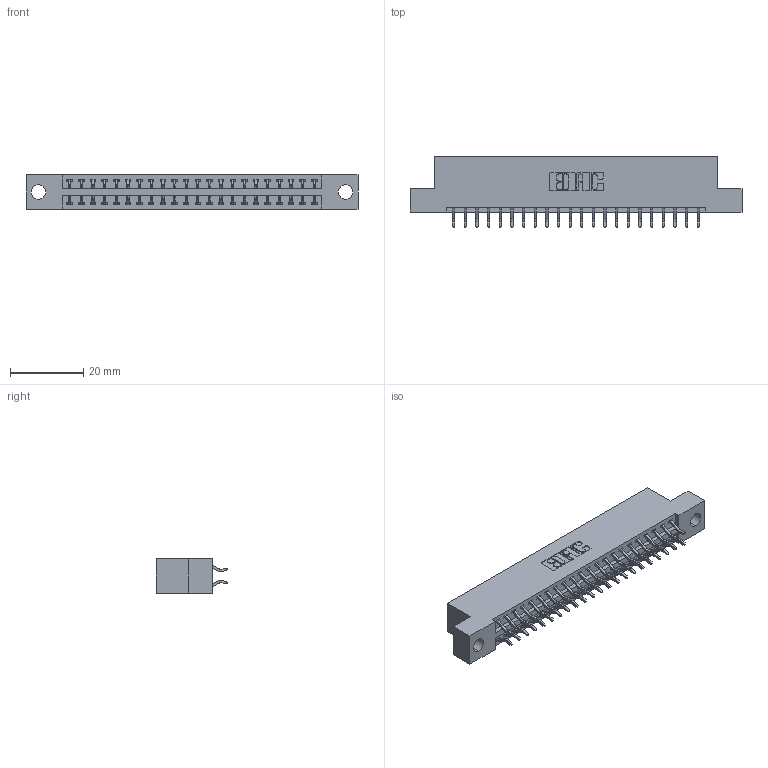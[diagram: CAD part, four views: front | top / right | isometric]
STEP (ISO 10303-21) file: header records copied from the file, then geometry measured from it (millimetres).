
FILE_DESCRIPTION (( 'STEP AP203' ), '1' );
FILE_NAME ('346-044-556-204.STEP', '2022-05-20T07:50:15', ( '' ), ( '' ), 'SwSTEP 2.0', 'SolidWorks 2020', '' );
FILE_SCHEMA (( 'CONFIG_CONTROL_DESIGN' ));
Length unit declared in the file: inch
Products named in the file (3): 345-292-001_556 Tail; 346-044-556-204; 346 Part_Flush Mounting Lugs - 0.156 Dia-TH
Assembly tree (45 placements, depth 2):
  346-044-556-204
    346 Part_Flush Mounting Lugs - 0.156 Dia-TH
    345-292-001_556 Tail  x44
Bounding box: 90.42 x 19.57 x 9.4 mm (x, y, z)
Volume: 8554.4 mm3; surface area: 11251.3 mm2
Topology: 45 solids, 45 shells, 2688 faces, 7977 edges, 5258 vertices
Faces by surface type: plane 1806, cylinder 882
Entity records: 17689 total; most frequent: CARTESIAN_POINT 2962, ORIENTED_EDGE 2882, DIRECTION 2649, EDGE_CURVE 1441, LINE 1213, VECTOR 1213, VERTEX_POINT 958, AXIS2_PLACEMENT_3D 718
